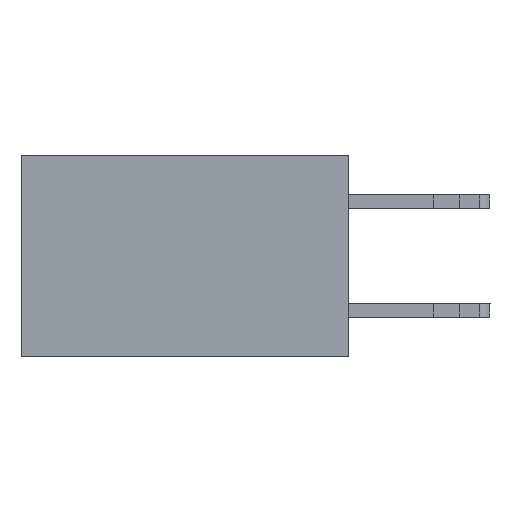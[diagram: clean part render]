
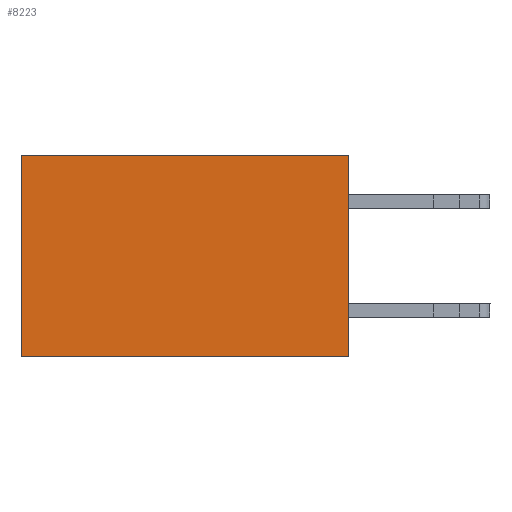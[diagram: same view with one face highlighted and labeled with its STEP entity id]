
A CAD part, left-side view. The second image highlights one B-rep face of the part: STEP entity #8223.
In plain terms, the highlighted planar face has unit normal (-1, 0, 0).
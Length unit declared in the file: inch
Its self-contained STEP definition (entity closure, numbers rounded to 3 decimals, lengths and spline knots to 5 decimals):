
#42 = DIRECTION ( 'NONE',  ( 0., 1., 0. ) ) ;
#98 = FACE_OUTER_BOUND ( 'NONE', #7001, .T. ) ;
#983 = CARTESIAN_POINT ( 'NONE',  ( 0.298, 0.6, -0.37 ) ) ;
#1089 = EDGE_CURVE ( 'NONE', #11342, #10809, #15053, .T. ) ;
#1798 = CARTESIAN_POINT ( 'NONE',  ( 0.298, 0.6, 0. ) ) ;
#1958 = DIRECTION ( 'NONE',  ( 0., 0., -1. ) ) ;
#2952 = AXIS2_PLACEMENT_3D ( 'NONE', #4298, #12084, #5979 ) ;
#3404 = ORIENTED_EDGE ( 'NONE', *, *, #12653, .F. ) ;
#3476 = CARTESIAN_POINT ( 'NONE',  ( 0.298, 0.6, 0. ) ) ;
#4298 = CARTESIAN_POINT ( 'NONE',  ( 0.298, 0., 0. ) ) ;
#4456 = CARTESIAN_POINT ( 'NONE',  ( 0.298, 0., -0.37 ) ) ;
#5979 = DIRECTION ( 'NONE',  ( 0., 0., -1. ) ) ;
#6460 = EDGE_CURVE ( 'NONE', #6564, #7555, #12703, .T. ) ;
#6564 = VERTEX_POINT ( 'NONE', #1798 ) ;
#6750 = CARTESIAN_POINT ( 'NONE',  ( 0.298, 0., -0.37 ) ) ;
#7001 = EDGE_LOOP ( 'NONE', ( #13060, #3404, #7421, #16073 ) ) ;
#7269 = PLANE ( 'NONE',  #2952 ) ;
#7421 = ORIENTED_EDGE ( 'NONE', *, *, #1089, .F. ) ;
#7555 = VERTEX_POINT ( 'NONE', #983 ) ;
#8223 = ADVANCED_FACE ( 'NONE', ( #98 ), #7269, .F. ) ;
#9560 = DIRECTION ( 'NONE',  ( 0., 0., -1. ) ) ;
#9562 = LINE ( 'NONE', #4456, #14629 ) ;
#10461 = VECTOR ( 'NONE', #9560, 39.37008 ) ;
#10551 = EDGE_CURVE ( 'NONE', #11342, #6564, #15457, .T. ) ;
#10809 = VERTEX_POINT ( 'NONE', #6750 ) ;
#10865 = VECTOR ( 'NONE', #42, 39.37008 ) ;
#11232 = VECTOR ( 'NONE', #1958, 39.37008 ) ;
#11342 = VERTEX_POINT ( 'NONE', #17270 ) ;
#12084 = DIRECTION ( 'NONE',  ( 1., 0., 0. ) ) ;
#12653 = EDGE_CURVE ( 'NONE', #10809, #7555, #9562, .T. ) ;
#12703 = LINE ( 'NONE', #3476, #11232 ) ;
#13060 = ORIENTED_EDGE ( 'NONE', *, *, #6460, .T. ) ;
#14629 = VECTOR ( 'NONE', #15251, 39.37008 ) ;
#15053 = LINE ( 'NONE', #17246, #10461 ) ;
#15251 = DIRECTION ( 'NONE',  ( 0., 1., 0. ) ) ;
#15457 = LINE ( 'NONE', #17858, #10865 ) ;
#16073 = ORIENTED_EDGE ( 'NONE', *, *, #10551, .T. ) ;
#17246 = CARTESIAN_POINT ( 'NONE',  ( 0.298, 0., 0. ) ) ;
#17270 = CARTESIAN_POINT ( 'NONE',  ( 0.298, 0., 0. ) ) ;
#17858 = CARTESIAN_POINT ( 'NONE',  ( 0.298, 0., 0. ) ) ;
